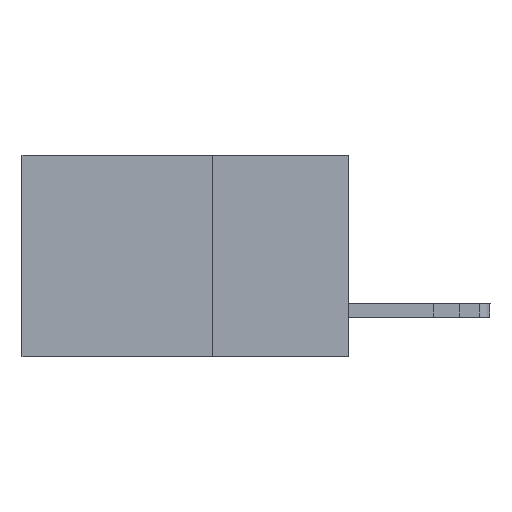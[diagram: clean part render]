
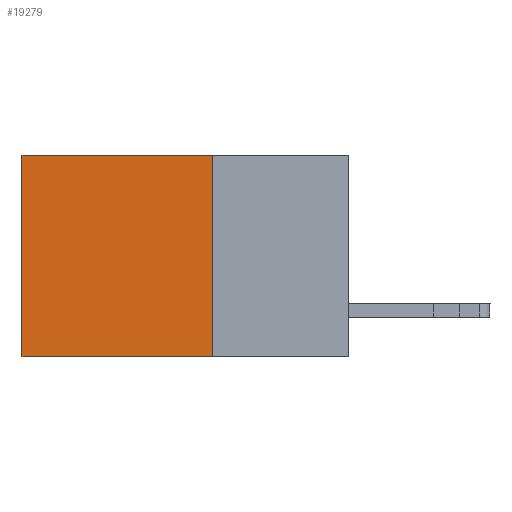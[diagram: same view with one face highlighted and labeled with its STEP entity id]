
A CAD part, left-side view. The second image highlights one B-rep face of the part: STEP entity #19279.
In plain terms, the highlighted planar face has unit normal (-1, 0, 0).
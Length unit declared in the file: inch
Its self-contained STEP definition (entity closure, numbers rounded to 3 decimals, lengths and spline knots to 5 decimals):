
#913 = EDGE_LOOP ( 'NONE', ( #2302, #13465, #7760, #14144 ) ) ;
#1150 = CARTESIAN_POINT ( 'NONE',  ( 0.2615, 0.25, -0.37 ) ) ;
#1152 = DIRECTION ( 'NONE',  ( 0., 0., -1. ) ) ;
#1417 = VERTEX_POINT ( 'NONE', #11515 ) ;
#2302 = ORIENTED_EDGE ( 'NONE', *, *, #12455, .T. ) ;
#2709 = LINE ( 'NONE', #6551, #14233 ) ;
#3145 = DIRECTION ( 'NONE',  ( 1., 0., 0. ) ) ;
#3873 = CARTESIAN_POINT ( 'NONE',  ( 0.2615, 0.25, 0. ) ) ;
#3971 = EDGE_CURVE ( 'NONE', #5465, #8934, #18511, .T. ) ;
#4342 = FACE_OUTER_BOUND ( 'NONE', #913, .T. ) ;
#4896 = AXIS2_PLACEMENT_3D ( 'NONE', #12245, #3145, #13676 ) ;
#5207 = VECTOR ( 'NONE', #8476, 39.37008 ) ;
#5465 = VERTEX_POINT ( 'NONE', #16210 ) ;
#5556 = CARTESIAN_POINT ( 'NONE',  ( 0.2615, 0.6, 0. ) ) ;
#6551 = CARTESIAN_POINT ( 'NONE',  ( 0.2615, 0.25, -0.37 ) ) ;
#6916 = VECTOR ( 'NONE', #1152, 39.37008 ) ;
#7760 = ORIENTED_EDGE ( 'NONE', *, *, #3971, .F. ) ;
#8100 = DIRECTION ( 'NONE',  ( 0., 1., 0. ) ) ;
#8476 = DIRECTION ( 'NONE',  ( 0., 1., 0. ) ) ;
#8934 = VERTEX_POINT ( 'NONE', #17678 ) ;
#11515 = CARTESIAN_POINT ( 'NONE',  ( 0.2615, 0.6, -0.37 ) ) ;
#12245 = CARTESIAN_POINT ( 'NONE',  ( 0.2615, 0.25, -0.37 ) ) ;
#12382 = EDGE_CURVE ( 'NONE', #8934, #1417, #2709, .T. ) ;
#12455 = EDGE_CURVE ( 'NONE', #17768, #1417, #17130, .T. ) ;
#13321 = EDGE_CURVE ( 'NONE', #5465, #17768, #16534, .T. ) ;
#13357 = VECTOR ( 'NONE', #15462, 39.37008 ) ;
#13465 = ORIENTED_EDGE ( 'NONE', *, *, #12382, .F. ) ;
#13676 = DIRECTION ( 'NONE',  ( 0., 0., -1. ) ) ;
#14144 = ORIENTED_EDGE ( 'NONE', *, *, #13321, .T. ) ;
#14233 = VECTOR ( 'NONE', #8100, 39.37008 ) ;
#15400 = CARTESIAN_POINT ( 'NONE',  ( 0.2615, 0.6, -0.37 ) ) ;
#15462 = DIRECTION ( 'NONE',  ( 0., 0., -1. ) ) ;
#16210 = CARTESIAN_POINT ( 'NONE',  ( 0.2615, 0.25, 0. ) ) ;
#16534 = LINE ( 'NONE', #3873, #5207 ) ;
#17130 = LINE ( 'NONE', #15400, #13357 ) ;
#17678 = CARTESIAN_POINT ( 'NONE',  ( 0.2615, 0.25, -0.37 ) ) ;
#17768 = VERTEX_POINT ( 'NONE', #5556 ) ;
#18511 = LINE ( 'NONE', #1150, #6916 ) ;
#19279 = ADVANCED_FACE ( 'NONE', ( #4342 ), #19316, .F. ) ;
#19316 = PLANE ( 'NONE',  #4896 ) ;
